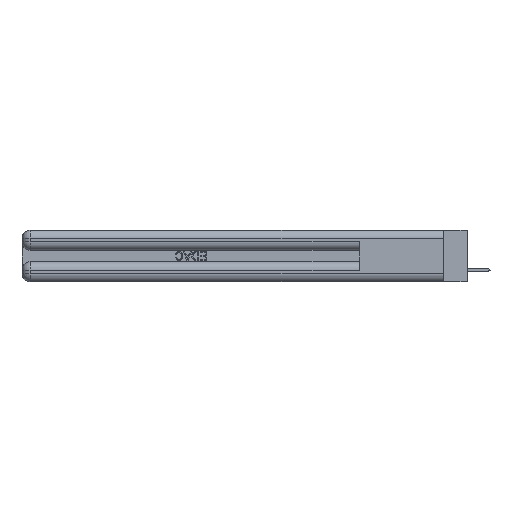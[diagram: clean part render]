
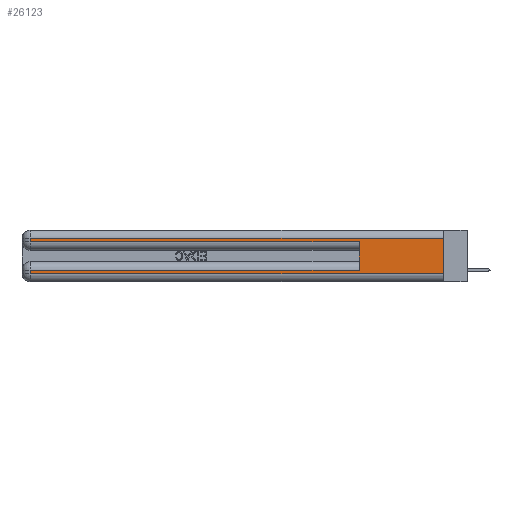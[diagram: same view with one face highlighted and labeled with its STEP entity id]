
A CAD part, left-side view. The second image highlights one B-rep face of the part: STEP entity #26123.
In plain terms, the highlighted planar face has unit normal (-1, 0, 0).
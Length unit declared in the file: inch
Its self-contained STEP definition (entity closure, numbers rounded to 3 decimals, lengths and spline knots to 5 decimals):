
#567 = CARTESIAN_POINT ( 'NONE',  ( 0., 2.94, 0.37 ) ) ;
#854 = CARTESIAN_POINT ( 'NONE',  ( 0., 0.6, 0.145 ) ) ;
#1203 = CARTESIAN_POINT ( 'NONE',  ( 0., 2.94, 0.37 ) ) ;
#1318 = CARTESIAN_POINT ( 'NONE',  ( 0., 0., 0.06 ) ) ;
#1384 = VERTEX_POINT ( 'NONE', #11069 ) ;
#2473 = CARTESIAN_POINT ( 'NONE',  ( 0., 0.6, 0.285 ) ) ;
#2776 = LINE ( 'NONE', #22340, #23200 ) ;
#3166 = VECTOR ( 'NONE', #36189, 39.37008 ) ;
#3247 = LINE ( 'NONE', #1318, #26474 ) ;
#3366 = LINE ( 'NONE', #1203, #19951 ) ;
#3439 = EDGE_CURVE ( 'NONE', #12737, #3787, #29597, .T. ) ;
#3787 = VERTEX_POINT ( 'NONE', #2473 ) ;
#4402 = DIRECTION ( 'NONE',  ( 0., 0., -1. ) ) ;
#5056 = ORIENTED_EDGE ( 'NONE', *, *, #19974, .T. ) ;
#5400 = CARTESIAN_POINT ( 'NONE',  ( 0., 0., 0.31 ) ) ;
#5880 = ORIENTED_EDGE ( 'NONE', *, *, #45646, .T. ) ;
#6236 = VERTEX_POINT ( 'NONE', #32360 ) ;
#7125 = ORIENTED_EDGE ( 'NONE', *, *, #29151, .T. ) ;
#8080 = VECTOR ( 'NONE', #37891, 39.37008 ) ;
#8932 = EDGE_CURVE ( 'NONE', #25148, #3787, #9251, .T. ) ;
#9251 = LINE ( 'NONE', #854, #3166 ) ;
#10627 = DIRECTION ( 'NONE',  ( 0., 0., -1. ) ) ;
#11069 = CARTESIAN_POINT ( 'NONE',  ( 0., 0., 0.06 ) ) ;
#12163 = DIRECTION ( 'NONE',  ( 0., 0., -1. ) ) ;
#12604 = DIRECTION ( 'NONE',  ( 0., -1., 0. ) ) ;
#12737 = VERTEX_POINT ( 'NONE', #30749 ) ;
#13070 = VECTOR ( 'NONE', #36444, 39.37008 ) ;
#13479 = CARTESIAN_POINT ( 'NONE',  ( 0., 2.94, 0.06 ) ) ;
#16454 = ORIENTED_EDGE ( 'NONE', *, *, #42719, .T. ) ;
#16633 = CARTESIAN_POINT ( 'NONE',  ( 0., 0., 0.085 ) ) ;
#19951 = VECTOR ( 'NONE', #12163, 39.37008 ) ;
#19974 = EDGE_CURVE ( 'NONE', #28765, #12737, #23586, .T. ) ;
#21234 = LINE ( 'NONE', #27867, #44330 ) ;
#22279 = AXIS2_PLACEMENT_3D ( 'NONE', #36184, #32179, #4402 ) ;
#22340 = CARTESIAN_POINT ( 'NONE',  ( 0., 0., 0.31 ) ) ;
#23200 = VECTOR ( 'NONE', #45677, 39.37008 ) ;
#23303 = ORIENTED_EDGE ( 'NONE', *, *, #8932, .F. ) ;
#23586 = LINE ( 'NONE', #567, #39050 ) ;
#24281 = VERTEX_POINT ( 'NONE', #13479 ) ;
#24580 = FACE_OUTER_BOUND ( 'NONE', #31820, .T. ) ;
#24901 = ORIENTED_EDGE ( 'NONE', *, *, #3439, .T. ) ;
#25148 = VERTEX_POINT ( 'NONE', #40048 ) ;
#26106 = EDGE_CURVE ( 'NONE', #37617, #1384, #21234, .T. ) ;
#26123 = ADVANCED_FACE ( 'NONE', ( #24580 ), #45497, .F. ) ;
#26474 = VECTOR ( 'NONE', #12604, 39.37008 ) ;
#27867 = CARTESIAN_POINT ( 'NONE',  ( 0., 0., 0.37 ) ) ;
#28368 = CARTESIAN_POINT ( 'NONE',  ( 0., 2.94, 0.31 ) ) ;
#28765 = VERTEX_POINT ( 'NONE', #28368 ) ;
#29151 = EDGE_CURVE ( 'NONE', #24281, #1384, #3247, .T. ) ;
#29597 = LINE ( 'NONE', #43178, #13070 ) ;
#29698 = ORIENTED_EDGE ( 'NONE', *, *, #26106, .F. ) ;
#30168 = LINE ( 'NONE', #16633, #8080 ) ;
#30361 = ORIENTED_EDGE ( 'NONE', *, *, #35176, .T. ) ;
#30749 = CARTESIAN_POINT ( 'NONE',  ( 0., 2.94, 0.285 ) ) ;
#31424 = DIRECTION ( 'NONE',  ( 0., 0., -1. ) ) ;
#31820 = EDGE_LOOP ( 'NONE', ( #29698, #16454, #5056, #24901, #23303, #5880, #30361, #7125 ) ) ;
#32179 = DIRECTION ( 'NONE',  ( 1., 0., 0. ) ) ;
#32360 = CARTESIAN_POINT ( 'NONE',  ( 0., 2.94, 0.085 ) ) ;
#35176 = EDGE_CURVE ( 'NONE', #6236, #24281, #3366, .T. ) ;
#36184 = CARTESIAN_POINT ( 'NONE',  ( 0., 0., 0.37 ) ) ;
#36189 = DIRECTION ( 'NONE',  ( 0., 0., 1. ) ) ;
#36444 = DIRECTION ( 'NONE',  ( 0., -1., 0. ) ) ;
#37617 = VERTEX_POINT ( 'NONE', #5400 ) ;
#37891 = DIRECTION ( 'NONE',  ( 0., 1., 0. ) ) ;
#39050 = VECTOR ( 'NONE', #10627, 39.37008 ) ;
#40048 = CARTESIAN_POINT ( 'NONE',  ( 0., 0.6, 0.085 ) ) ;
#42719 = EDGE_CURVE ( 'NONE', #37617, #28765, #2776, .T. ) ;
#43178 = CARTESIAN_POINT ( 'NONE',  ( 0., 0., 0.285 ) ) ;
#44330 = VECTOR ( 'NONE', #31424, 39.37008 ) ;
#45497 = PLANE ( 'NONE',  #22279 ) ;
#45646 = EDGE_CURVE ( 'NONE', #25148, #6236, #30168, .T. ) ;
#45677 = DIRECTION ( 'NONE',  ( 0., 1., 0. ) ) ;
